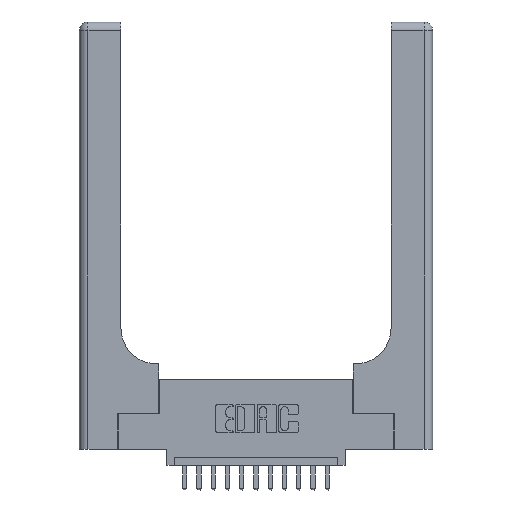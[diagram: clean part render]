
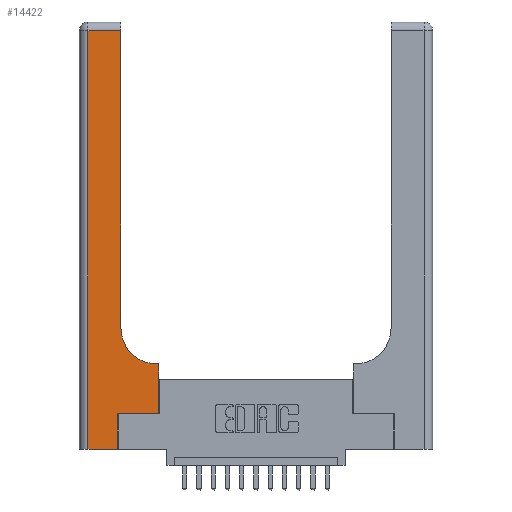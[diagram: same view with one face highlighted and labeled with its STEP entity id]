
A CAD part, top view. The second image highlights one B-rep face of the part: STEP entity #14422.
In plain terms, the highlighted planar face has unit normal (0, 0, 1).
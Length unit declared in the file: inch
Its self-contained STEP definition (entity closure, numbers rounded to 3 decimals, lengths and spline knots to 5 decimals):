
#1021 = VECTOR ( 'NONE', #4805, 39.37008 ) ;
#1041 = LINE ( 'NONE', #7917, #15281 ) ;
#1127 = LINE ( 'NONE', #14705, #17758 ) ;
#1199 = EDGE_LOOP ( 'NONE', ( #10074, #2503, #15983, #17726, #16598, #9325, #11155, #4674, #1481 ) ) ;
#1387 = CARTESIAN_POINT ( 'NONE',  ( 0.06, 2.94, 0.37 ) ) ;
#1481 = ORIENTED_EDGE ( 'NONE', *, *, #5610, .T. ) ;
#1799 = CARTESIAN_POINT ( 'NONE',  ( 0.5585, 0.6, 0.37 ) ) ;
#1875 = DIRECTION ( 'NONE',  ( 1., 0., 0. ) ) ;
#2296 = CARTESIAN_POINT ( 'NONE',  ( 0.2915, 0.6, 0.37 ) ) ;
#2503 = ORIENTED_EDGE ( 'NONE', *, *, #4487, .T. ) ;
#2586 = CARTESIAN_POINT ( 'NONE',  ( 0.269, 0.25, 0.37 ) ) ;
#2647 = EDGE_CURVE ( 'NONE', #5572, #7395, #1041, .T. ) ;
#2728 = DIRECTION ( 'NONE',  ( -1., 0., 0. ) ) ;
#2967 = VERTEX_POINT ( 'NONE', #7052 ) ;
#3163 = PLANE ( 'NONE',  #13164 ) ;
#3384 = VECTOR ( 'NONE', #3679, 39.37008 ) ;
#3679 = DIRECTION ( 'NONE',  ( -1., 0., 0. ) ) ;
#4487 = EDGE_CURVE ( 'NONE', #4717, #13551, #8362, .T. ) ;
#4545 = DIRECTION ( 'NONE',  ( 0., 0., -1. ) ) ;
#4674 = ORIENTED_EDGE ( 'NONE', *, *, #17806, .T. ) ;
#4717 = VERTEX_POINT ( 'NONE', #5897 ) ;
#4805 = DIRECTION ( 'NONE',  ( 0., 1., 0. ) ) ;
#5249 = LINE ( 'NONE', #2586, #17077 ) ;
#5572 = VERTEX_POINT ( 'NONE', #15016 ) ;
#5610 = EDGE_CURVE ( 'NONE', #15815, #2967, #15863, .T. ) ;
#5897 = CARTESIAN_POINT ( 'NONE',  ( 0.2915, 2.94, 0.37 ) ) ;
#5926 = DIRECTION ( 'NONE',  ( -1., 0., 0. ) ) ;
#6099 = CARTESIAN_POINT ( 'NONE',  ( 0.269, 0.25, 0.37 ) ) ;
#6119 = CARTESIAN_POINT ( 'NONE',  ( 0., 3., 0.37 ) ) ;
#7026 = EDGE_CURVE ( 'NONE', #11484, #5572, #5249, .T. ) ;
#7029 = CARTESIAN_POINT ( 'NONE',  ( 0.5415, 0.6, 0.37 ) ) ;
#7052 = CARTESIAN_POINT ( 'NONE',  ( 0.2915, 0.85, 0.37 ) ) ;
#7395 = VERTEX_POINT ( 'NONE', #1799 ) ;
#7782 = EDGE_CURVE ( 'NONE', #11383, #11484, #15472, .T. ) ;
#7917 = CARTESIAN_POINT ( 'NONE',  ( 0.5585, 0.25, 0.37 ) ) ;
#7982 = DIRECTION ( 'NONE',  ( 0., 1., 0. ) ) ;
#8133 = DIRECTION ( 'NONE',  ( 0., -1., 0. ) ) ;
#8148 = CARTESIAN_POINT ( 'NONE',  ( 0.5415, 0.85, 0.37 ) ) ;
#8348 = EDGE_CURVE ( 'NONE', #13551, #11500, #17838, .T. ) ;
#8362 = LINE ( 'NONE', #17473, #3384 ) ;
#8539 = CARTESIAN_POINT ( 'NONE',  ( 0.269, 0., 0.37 ) ) ;
#8926 = CARTESIAN_POINT ( 'NONE',  ( 0.269, 0., 0.37 ) ) ;
#9325 = ORIENTED_EDGE ( 'NONE', *, *, #7026, .T. ) ;
#9383 = EDGE_CURVE ( 'NONE', #11500, #11383, #17571, .T. ) ;
#10074 = ORIENTED_EDGE ( 'NONE', *, *, #10617, .T. ) ;
#10380 = CARTESIAN_POINT ( 'NONE',  ( 0., 0., 0.37 ) ) ;
#10416 = FACE_OUTER_BOUND ( 'NONE', #1199, .T. ) ;
#10527 = VECTOR ( 'NONE', #2728, 39.37008 ) ;
#10617 = EDGE_CURVE ( 'NONE', #2967, #4717, #1127, .T. ) ;
#11155 = ORIENTED_EDGE ( 'NONE', *, *, #2647, .T. ) ;
#11383 = VERTEX_POINT ( 'NONE', #8539 ) ;
#11484 = VERTEX_POINT ( 'NONE', #6099 ) ;
#11500 = VERTEX_POINT ( 'NONE', #11622 ) ;
#11622 = CARTESIAN_POINT ( 'NONE',  ( 0.06, 0., 0.37 ) ) ;
#12094 = DIRECTION ( 'NONE',  ( 0., 1., 0. ) ) ;
#12197 = DIRECTION ( 'NONE',  ( 0., 0., -1. ) ) ;
#13014 = CARTESIAN_POINT ( 'NONE',  ( 0.06, 3., 0.37 ) ) ;
#13164 = AXIS2_PLACEMENT_3D ( 'NONE', #6119, #4545, #5926 ) ;
#13551 = VERTEX_POINT ( 'NONE', #1387 ) ;
#14122 = VECTOR ( 'NONE', #8133, 39.37008 ) ;
#14422 = ADVANCED_FACE ( 'NONE', ( #10416 ), #3163, .F. ) ;
#14705 = CARTESIAN_POINT ( 'NONE',  ( 0.2915, 3., 0.37 ) ) ;
#15016 = CARTESIAN_POINT ( 'NONE',  ( 0.5585, 0.25, 0.37 ) ) ;
#15281 = VECTOR ( 'NONE', #7982, 39.37008 ) ;
#15472 = LINE ( 'NONE', #8926, #1021 ) ;
#15540 = AXIS2_PLACEMENT_3D ( 'NONE', #8148, #12197, #17835 ) ;
#15574 = DIRECTION ( 'NONE',  ( 1., 0., 0. ) ) ;
#15815 = VERTEX_POINT ( 'NONE', #7029 ) ;
#15863 = CIRCLE ( 'NONE', #15540, 0.25 ) ;
#15983 = ORIENTED_EDGE ( 'NONE', *, *, #8348, .T. ) ;
#16081 = VECTOR ( 'NONE', #1875, 39.37008 ) ;
#16171 = LINE ( 'NONE', #2296, #10527 ) ;
#16598 = ORIENTED_EDGE ( 'NONE', *, *, #7782, .T. ) ;
#17077 = VECTOR ( 'NONE', #15574, 39.37008 ) ;
#17473 = CARTESIAN_POINT ( 'NONE',  ( 0., 2.94, 0.37 ) ) ;
#17571 = LINE ( 'NONE', #10380, #16081 ) ;
#17726 = ORIENTED_EDGE ( 'NONE', *, *, #9383, .T. ) ;
#17758 = VECTOR ( 'NONE', #12094, 39.37008 ) ;
#17806 = EDGE_CURVE ( 'NONE', #7395, #15815, #16171, .T. ) ;
#17835 = DIRECTION ( 'NONE',  ( 1., 0., 0. ) ) ;
#17838 = LINE ( 'NONE', #13014, #14122 ) ;
